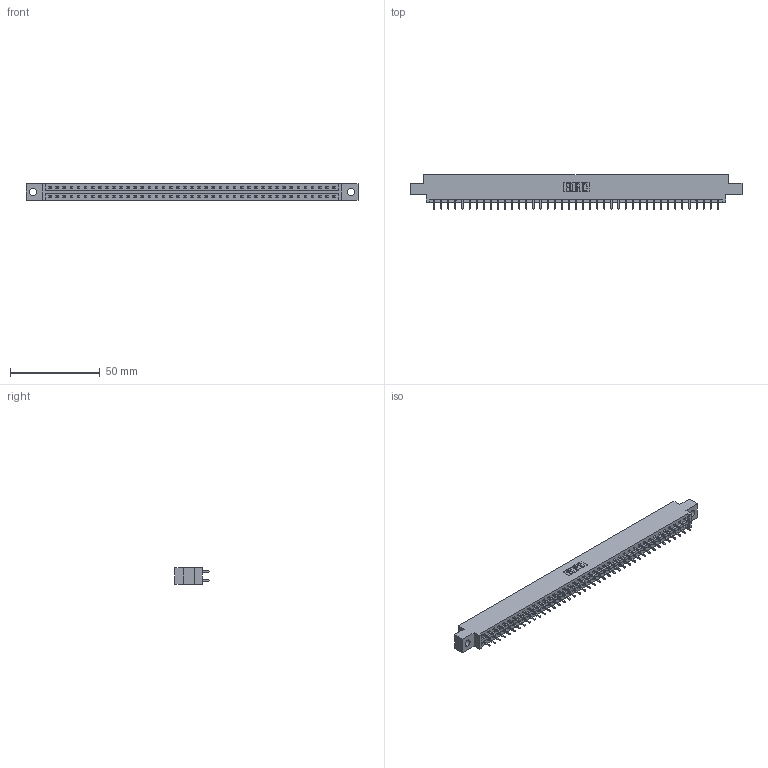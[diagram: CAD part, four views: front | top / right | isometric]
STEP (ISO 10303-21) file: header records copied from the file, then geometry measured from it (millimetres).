
FILE_DESCRIPTION (( 'STEP AP203' ), '1' );
FILE_NAME ('337-082-521-804.STEP', '2019-10-15T16:05:49', ( '' ), ( '' ), 'SwSTEP 2.0', 'SolidWorks 2016', '' );
FILE_SCHEMA (( 'CONFIG_CONTROL_DESIGN' ));
Length unit declared in the file: inch
Products named in the file (3): 337 Part_0.170 Offset - 0.156 Dia-TH; 345-292-001_345-293-121; 337-082-521-804
Assembly tree (83 placements, depth 2):
  337-082-521-804
    337 Part_0.170 Offset - 0.156 Dia-TH
    345-292-001_345-293-121  x82
Bounding box: 185.47 x 19.06 x 9.4 mm (x, y, z)
Volume: 19294.2 mm3; surface area: 21464.6 mm2
Topology: 83 solids, 83 shells, 4546 faces, 13525 edges, 8906 vertices
Faces by surface type: plane 3190, cylinder 1356
Entity records: 32071 total; most frequent: CARTESIAN_POINT 5406, ORIENTED_EDGE 5342, DIRECTION 4599, EDGE_CURVE 2671, VECTOR 2543, LINE 2543, VERTEX_POINT 1778, AXIS2_PLACEMENT_3D 1028
